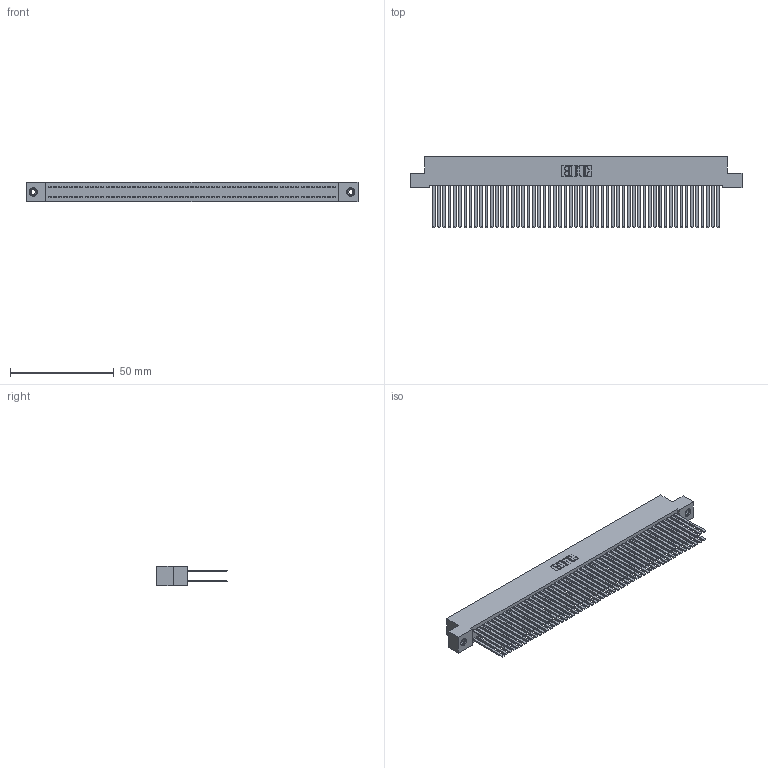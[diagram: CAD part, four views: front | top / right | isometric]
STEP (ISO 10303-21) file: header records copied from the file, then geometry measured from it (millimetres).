
FILE_DESCRIPTION (( 'STEP AP203' ), '1' );
FILE_NAME ('392-110-544-208.STEP', '2019-10-09T23:53:52', ( '' ), ( '' ), 'SwSTEP 2.0', 'SolidWorks 2016', '' );
FILE_SCHEMA (( 'CONFIG_CONTROL_DESIGN' ));
Length unit declared in the file: inch
Products named in the file (4): 342 Part_TI; 345-292-001_345-293-144; 345-250-001_345-250-003-102; 392-110-544-208
Assembly tree (113 placements, depth 2):
  392-110-544-208
    342 Part_TI
    345-292-001_345-293-144  x110
    345-250-001_345-250-003-102  x2
Bounding box: 160.02 x 34.3 x 9.4 mm (x, y, z)
Volume: 15975.6 mm3; surface area: 30605.3 mm2
Topology: 113 solids, 113 shells, 5230 faces, 15505 edges, 10182 vertices
Faces by surface type: plane 3618, cylinder 1596, cone 12, torus 4
Entity records: 34572 total; most frequent: CARTESIAN_POINT 5693, ORIENTED_EDGE 5622, DIRECTION 4869, EDGE_CURVE 2811, LINE 2667, VECTOR 2667, VERTEX_POINT 1868, AXIS2_PLACEMENT_3D 1101
